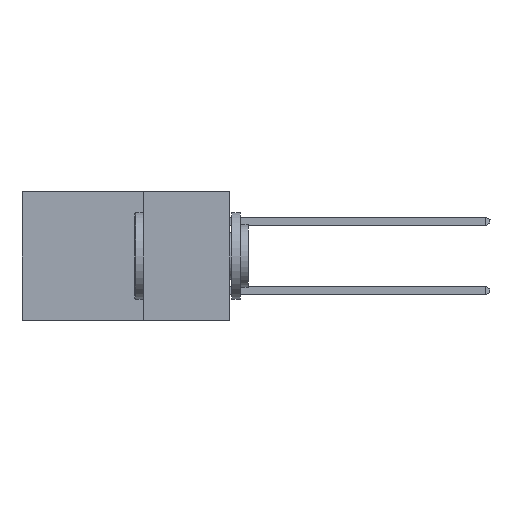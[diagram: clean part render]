
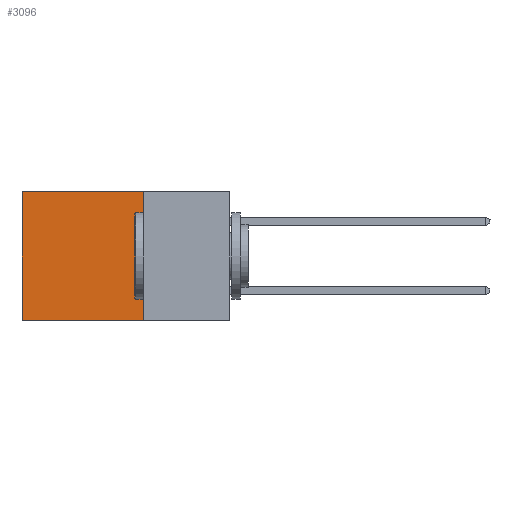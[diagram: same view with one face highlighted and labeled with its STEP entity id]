
A CAD part, left-side view. The second image highlights one B-rep face of the part: STEP entity #3096.
In plain terms, the highlighted planar face has unit normal (-1, 0, 0).
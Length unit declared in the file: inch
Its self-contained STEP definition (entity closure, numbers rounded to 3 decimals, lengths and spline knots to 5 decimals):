
#459 = VECTOR ( 'NONE', #9632, 39.37008 ) ;
#623 = VERTEX_POINT ( 'NONE', #2998 ) ;
#1312 = CARTESIAN_POINT ( 'NONE',  ( 0.2615, 0.25, 0. ) ) ;
#1427 = ORIENTED_EDGE ( 'NONE', *, *, #10325, .T. ) ;
#1872 = VERTEX_POINT ( 'NONE', #5135 ) ;
#2257 = FACE_OUTER_BOUND ( 'NONE', #5240, .T. ) ;
#2397 = EDGE_CURVE ( 'NONE', #623, #8997, #9097, .T. ) ;
#2818 = CARTESIAN_POINT ( 'NONE',  ( 0.2615, 0.6, -0.37 ) ) ;
#2998 = CARTESIAN_POINT ( 'NONE',  ( 0.2615, 0.25, -0.37 ) ) ;
#3096 = ADVANCED_FACE ( 'NONE', ( #2257 ), #5537, .F. ) ;
#3513 = VECTOR ( 'NONE', #6866, 39.37008 ) ;
#3655 = ORIENTED_EDGE ( 'NONE', *, *, #8996, .T. ) ;
#3811 = DIRECTION ( 'NONE',  ( 0., 0., -1. ) ) ;
#3917 = DIRECTION ( 'NONE',  ( 0., 0., -1. ) ) ;
#4154 = CARTESIAN_POINT ( 'NONE',  ( 0.2615, 0.25, -0.37 ) ) ;
#5135 = CARTESIAN_POINT ( 'NONE',  ( 0.2615, 0.6, 0. ) ) ;
#5240 = EDGE_LOOP ( 'NONE', ( #1427, #5309, #10396, #3655 ) ) ;
#5309 = ORIENTED_EDGE ( 'NONE', *, *, #2397, .F. ) ;
#5389 = CARTESIAN_POINT ( 'NONE',  ( 0.2615, 0.6, -0.37 ) ) ;
#5480 = DIRECTION ( 'NONE',  ( 1., 0., 0. ) ) ;
#5537 = PLANE ( 'NONE',  #8252 ) ;
#6225 = LINE ( 'NONE', #8068, #8097 ) ;
#6747 = CARTESIAN_POINT ( 'NONE',  ( 0.2615, 0.25, 0. ) ) ;
#6866 = DIRECTION ( 'NONE',  ( 0., 1., 0. ) ) ;
#8068 = CARTESIAN_POINT ( 'NONE',  ( 0.2615, 0.25, -0.37 ) ) ;
#8097 = VECTOR ( 'NONE', #3917, 39.37008 ) ;
#8252 = AXIS2_PLACEMENT_3D ( 'NONE', #9013, #5480, #9769 ) ;
#8526 = EDGE_CURVE ( 'NONE', #9245, #623, #6225, .T. ) ;
#8996 = EDGE_CURVE ( 'NONE', #9245, #1872, #9471, .T. ) ;
#8997 = VERTEX_POINT ( 'NONE', #2818 ) ;
#9013 = CARTESIAN_POINT ( 'NONE',  ( 0.2615, 0.25, -0.37 ) ) ;
#9097 = LINE ( 'NONE', #4154, #3513 ) ;
#9245 = VERTEX_POINT ( 'NONE', #6747 ) ;
#9471 = LINE ( 'NONE', #1312, #459 ) ;
#9632 = DIRECTION ( 'NONE',  ( 0., 1., 0. ) ) ;
#9769 = DIRECTION ( 'NONE',  ( 0., 0., -1. ) ) ;
#10007 = VECTOR ( 'NONE', #3811, 39.37008 ) ;
#10325 = EDGE_CURVE ( 'NONE', #1872, #8997, #10445, .T. ) ;
#10396 = ORIENTED_EDGE ( 'NONE', *, *, #8526, .F. ) ;
#10445 = LINE ( 'NONE', #5389, #10007 ) ;
